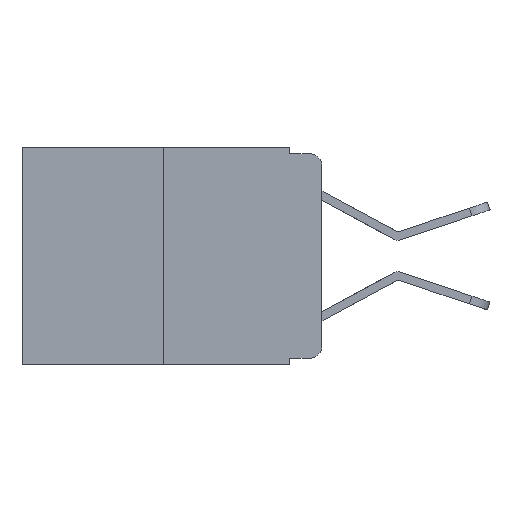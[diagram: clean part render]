
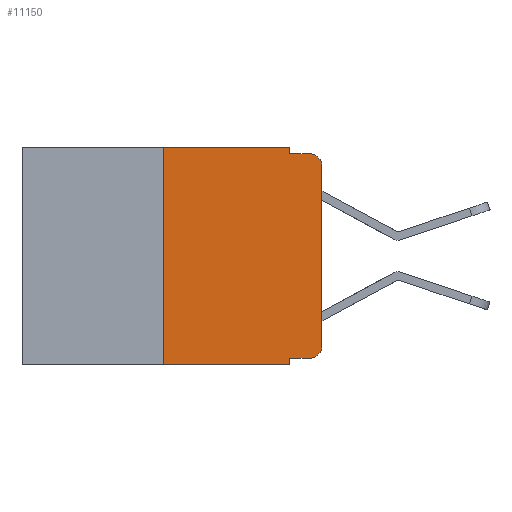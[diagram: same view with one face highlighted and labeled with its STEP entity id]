
A CAD part, left-side view. The second image highlights one B-rep face of the part: STEP entity #11150.
In plain terms, the highlighted planar face has unit normal (-1, 0, 0).
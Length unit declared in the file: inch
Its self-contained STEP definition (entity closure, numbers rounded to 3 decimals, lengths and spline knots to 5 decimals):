
#97 = CARTESIAN_POINT ( 'NONE',  ( 0., 0., -0.313 ) ) ;
#206 = CARTESIAN_POINT ( 'NONE',  ( 0., 0.473, -0.343 ) ) ;
#369 = ORIENTED_EDGE ( 'NONE', *, *, #15253, .F. ) ;
#597 = CIRCLE ( 'NONE', #985, 0.02 ) ;
#685 = LINE ( 'NONE', #12653, #12998 ) ;
#985 = AXIS2_PLACEMENT_3D ( 'NONE', #8266, #11023, #15077 ) ;
#1070 = EDGE_CURVE ( 'NONE', #5005, #14564, #685, .T. ) ;
#1193 = DIRECTION ( 'NONE',  ( 0., 0., 1. ) ) ;
#1303 = EDGE_CURVE ( 'NONE', #14259, #2273, #16836, .T. ) ;
#1466 = DIRECTION ( 'NONE',  ( 0., -1., 0. ) ) ;
#1843 = DIRECTION ( 'NONE',  ( -1., 0., 0. ) ) ;
#2271 = CARTESIAN_POINT ( 'NONE',  ( 0., 0.051, -0.01 ) ) ;
#2273 = VERTEX_POINT ( 'NONE', #5599 ) ;
#2761 = CARTESIAN_POINT ( 'NONE',  ( 0., 0.25, 0. ) ) ;
#3473 = VERTEX_POINT ( 'NONE', #97 ) ;
#3671 = LINE ( 'NONE', #206, #4091 ) ;
#3752 = ORIENTED_EDGE ( 'NONE', *, *, #7315, .F. ) ;
#4085 = CARTESIAN_POINT ( 'NONE',  ( 0., 0.473, 0. ) ) ;
#4091 = VECTOR ( 'NONE', #4263, 39.37008 ) ;
#4226 = VECTOR ( 'NONE', #16586, 39.37008 ) ;
#4263 = DIRECTION ( 'NONE',  ( 0., -1., 0. ) ) ;
#4288 = CARTESIAN_POINT ( 'NONE',  ( 0., 0.051, 0. ) ) ;
#4469 = DIRECTION ( 'NONE',  ( 0., 0., 1. ) ) ;
#4611 = VERTEX_POINT ( 'NONE', #10734 ) ;
#4627 = AXIS2_PLACEMENT_3D ( 'NONE', #15581, #13377, #6501 ) ;
#4764 = CARTESIAN_POINT ( 'NONE',  ( 0., 0.051, 0. ) ) ;
#4792 = VECTOR ( 'NONE', #7727, 39.37008 ) ;
#5005 = VERTEX_POINT ( 'NONE', #12808 ) ;
#5487 = FACE_OUTER_BOUND ( 'NONE', #10927, .T. ) ;
#5599 = CARTESIAN_POINT ( 'NONE',  ( 0., 0.051, -0.343 ) ) ;
#6159 = EDGE_CURVE ( 'NONE', #11694, #3473, #597, .T. ) ;
#6501 = DIRECTION ( 'NONE',  ( 0., 0., -1. ) ) ;
#6569 = CARTESIAN_POINT ( 'NONE',  ( 0., 0.051, -0.333 ) ) ;
#7272 = CARTESIAN_POINT ( 'NONE',  ( 0., 0.02, -0.333 ) ) ;
#7315 = EDGE_CURVE ( 'NONE', #9331, #16164, #9921, .T. ) ;
#7578 = LINE ( 'NONE', #2271, #4792 ) ;
#7619 = ORIENTED_EDGE ( 'NONE', *, *, #9890, .T. ) ;
#7727 = DIRECTION ( 'NONE',  ( 0., -1., 0. ) ) ;
#8168 = EDGE_CURVE ( 'NONE', #5005, #2273, #3671, .T. ) ;
#8232 = ORIENTED_EDGE ( 'NONE', *, *, #16669, .F. ) ;
#8266 = CARTESIAN_POINT ( 'NONE',  ( 0., 0.02, -0.313 ) ) ;
#8825 = EDGE_CURVE ( 'NONE', #14259, #11694, #10910, .T. ) ;
#8873 = CARTESIAN_POINT ( 'NONE',  ( 0., 0.051, 0. ) ) ;
#9290 = ORIENTED_EDGE ( 'NONE', *, *, #8825, .T. ) ;
#9331 = VERTEX_POINT ( 'NONE', #8873 ) ;
#9372 = DIRECTION ( 'NONE',  ( 0., -1., 0. ) ) ;
#9437 = VECTOR ( 'NONE', #1466, 39.37008 ) ;
#9636 = VECTOR ( 'NONE', #9372, 39.37008 ) ;
#9831 = CARTESIAN_POINT ( 'NONE',  ( 0., 0.02, -0.01 ) ) ;
#9838 = VECTOR ( 'NONE', #1193, 39.37008 ) ;
#9890 = EDGE_CURVE ( 'NONE', #3473, #4611, #13462, .T. ) ;
#9921 = LINE ( 'NONE', #4764, #10356 ) ;
#10015 = ORIENTED_EDGE ( 'NONE', *, *, #1070, .F. ) ;
#10086 = LINE ( 'NONE', #4085, #9437 ) ;
#10356 = VECTOR ( 'NONE', #10627, 39.37008 ) ;
#10501 = ORIENTED_EDGE ( 'NONE', *, *, #12855, .T. ) ;
#10627 = DIRECTION ( 'NONE',  ( 0., 0., -1. ) ) ;
#10734 = CARTESIAN_POINT ( 'NONE',  ( 0., 0., -0.03 ) ) ;
#10910 = LINE ( 'NONE', #6569, #9636 ) ;
#10927 = EDGE_LOOP ( 'NONE', ( #7619, #10501, #8232, #3752, #369, #10015, #11803, #13554, #9290, #12416 ) ) ;
#11023 = DIRECTION ( 'NONE',  ( -1., 0., 0. ) ) ;
#11150 = ADVANCED_FACE ( 'NONE', ( #5487 ), #17145, .F. ) ;
#11694 = VERTEX_POINT ( 'NONE', #7272 ) ;
#11771 = CARTESIAN_POINT ( 'NONE',  ( 0., 0.051, -0.333 ) ) ;
#11803 = ORIENTED_EDGE ( 'NONE', *, *, #8168, .T. ) ;
#12241 = VERTEX_POINT ( 'NONE', #9831 ) ;
#12416 = ORIENTED_EDGE ( 'NONE', *, *, #6159, .T. ) ;
#12653 = CARTESIAN_POINT ( 'NONE',  ( 0., 0.25, 0. ) ) ;
#12808 = CARTESIAN_POINT ( 'NONE',  ( 0., 0.25, -0.343 ) ) ;
#12855 = EDGE_CURVE ( 'NONE', #4611, #12241, #13368, .T. ) ;
#12998 = VECTOR ( 'NONE', #4469, 39.37008 ) ;
#13204 = CARTESIAN_POINT ( 'NONE',  ( 0., 0., 0. ) ) ;
#13368 = CIRCLE ( 'NONE', #15058, 0.02 ) ;
#13377 = DIRECTION ( 'NONE',  ( 1., 0., 0. ) ) ;
#13462 = LINE ( 'NONE', #13204, #9838 ) ;
#13554 = ORIENTED_EDGE ( 'NONE', *, *, #1303, .F. ) ;
#14259 = VERTEX_POINT ( 'NONE', #11771 ) ;
#14564 = VERTEX_POINT ( 'NONE', #2761 ) ;
#15058 = AXIS2_PLACEMENT_3D ( 'NONE', #15453, #1843, #16713 ) ;
#15077 = DIRECTION ( 'NONE',  ( 0., 0., -1. ) ) ;
#15253 = EDGE_CURVE ( 'NONE', #14564, #9331, #10086, .T. ) ;
#15453 = CARTESIAN_POINT ( 'NONE',  ( 0., 0.02, -0.03 ) ) ;
#15581 = CARTESIAN_POINT ( 'NONE',  ( 0., 0.473, 0. ) ) ;
#16164 = VERTEX_POINT ( 'NONE', #17505 ) ;
#16586 = DIRECTION ( 'NONE',  ( 0., 0., -1. ) ) ;
#16669 = EDGE_CURVE ( 'NONE', #16164, #12241, #7578, .T. ) ;
#16713 = DIRECTION ( 'NONE',  ( 0., 0., -1. ) ) ;
#16836 = LINE ( 'NONE', #4288, #4226 ) ;
#17145 = PLANE ( 'NONE',  #4627 ) ;
#17505 = CARTESIAN_POINT ( 'NONE',  ( 0., 0.051, -0.01 ) ) ;
